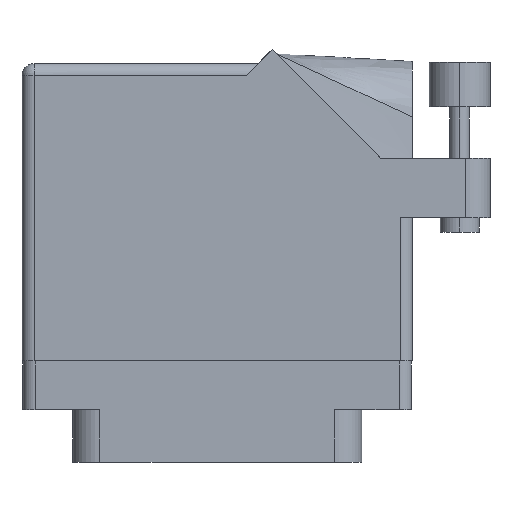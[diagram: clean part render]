
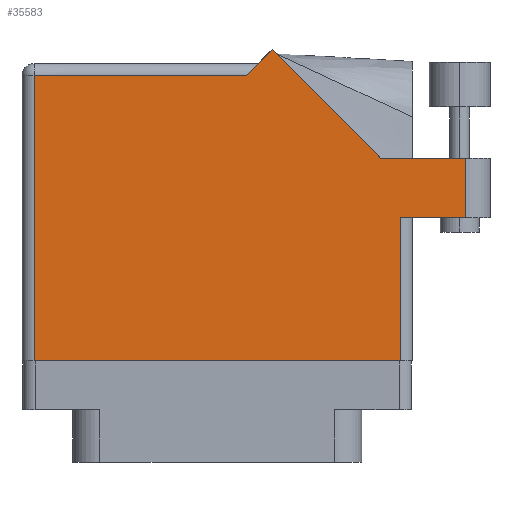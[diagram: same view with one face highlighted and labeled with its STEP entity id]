
A CAD part, front view. The second image highlights one B-rep face of the part: STEP entity #35583.
In plain terms, the highlighted face is planar.
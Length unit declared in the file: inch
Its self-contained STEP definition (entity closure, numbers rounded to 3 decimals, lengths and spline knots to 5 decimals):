
#87 = DIRECTION ( 'NONE',  ( -1., 0., 0. ) ) ;
#300 = LINE ( 'NONE', #7329, #24097 ) ;
#316 = DIRECTION ( 'NONE',  ( 1., 0., 0. ) ) ;
#977 = PLANE ( 'NONE',  #6556 ) ;
#1497 = LINE ( 'NONE', #14227, #21332 ) ;
#1553 = LINE ( 'NONE', #28286, #30628 ) ;
#1587 = EDGE_CURVE ( 'NONE', #17479, #24316, #30932, .T. ) ;
#1897 = ORIENTED_EDGE ( 'NONE', *, *, #10935, .T. ) ;
#1936 = ORIENTED_EDGE ( 'NONE', *, *, #35250, .T. ) ;
#4389 = VECTOR ( 'NONE', #36227, 39.37008 ) ;
#5711 = CARTESIAN_POINT ( 'NONE',  ( 0.83942, 0.944, 0.455 ) ) ;
#5885 = LINE ( 'NONE', #14596, #4389 ) ;
#6556 = AXIS2_PLACEMENT_3D ( 'NONE', #22632, #25769, #38970 ) ;
#7041 = EDGE_CURVE ( 'NONE', #25295, #24932, #35793, .T. ) ;
#7329 = CARTESIAN_POINT ( 'NONE',  ( 1.405, 0.944, 0.455 ) ) ;
#8422 = ORIENTED_EDGE ( 'NONE', *, *, #7041, .T. ) ;
#8563 = LINE ( 'NONE', #26989, #35157 ) ;
#9978 = ORIENTED_EDGE ( 'NONE', *, *, #16870, .T. ) ;
#10122 = ORIENTED_EDGE ( 'NONE', *, *, #39444, .T. ) ;
#10469 = FACE_OUTER_BOUND ( 'NONE', #15278, .T. ) ;
#10810 = DIRECTION ( 'NONE',  ( -0.707, 0.707, 0. ) ) ;
#10935 = EDGE_CURVE ( 'NONE', #15507, #30508, #1553, .T. ) ;
#11664 = CARTESIAN_POINT ( 'NONE',  ( 1.28, 0.637, 0.455 ) ) ;
#11964 = LINE ( 'NONE', #18461, #35651 ) ;
#12001 = DIRECTION ( 'NONE',  ( 0., 1., 0. ) ) ;
#12781 = CARTESIAN_POINT ( 'NONE',  ( 0.943, 0.637, 0.455 ) ) ;
#13068 = VECTOR ( 'NONE', #87, 39.37008 ) ;
#13102 = ORIENTED_EDGE ( 'NONE', *, *, #14538, .T. ) ;
#13276 = CARTESIAN_POINT ( 'NONE',  ( 0.28271, 1.50071, 0.455 ) ) ;
#14227 = CARTESIAN_POINT ( 'NONE',  ( -0.943, -0.1, 0.455 ) ) ;
#14538 = EDGE_CURVE ( 'NONE', #24932, #17479, #1497, .T. ) ;
#14596 = CARTESIAN_POINT ( 'NONE',  ( 0.212, 1.43, 0.455 ) ) ;
#14768 = DIRECTION ( 'NONE',  ( 0., -1., 0. ) ) ;
#15278 = EDGE_LOOP ( 'NONE', ( #39815, #1897, #9978, #10122, #18293, #8422, #13102, #37050, #1936 ) ) ;
#15507 = VERTEX_POINT ( 'NONE', #11664 ) ;
#16870 = EDGE_CURVE ( 'NONE', #30508, #20123, #300, .T. ) ;
#17025 = EDGE_CURVE ( 'NONE', #35901, #25295, #5885, .T. ) ;
#17479 = VERTEX_POINT ( 'NONE', #33991 ) ;
#17503 = DIRECTION ( 'NONE',  ( 1., 0., 0. ) ) ;
#18293 = ORIENTED_EDGE ( 'NONE', *, *, #17025, .T. ) ;
#18461 = CARTESIAN_POINT ( 'NONE',  ( 0.943, 0.637, 0.455 ) ) ;
#18720 = CARTESIAN_POINT ( 'NONE',  ( -0.943, 1.368, 0.455 ) ) ;
#20123 = VERTEX_POINT ( 'NONE', #5711 ) ;
#20669 = LINE ( 'NONE', #38901, #37548 ) ;
#21332 = VECTOR ( 'NONE', #14768, 39.37008 ) ;
#21971 = CARTESIAN_POINT ( 'NONE',  ( -1.005, -0.1, 0.455 ) ) ;
#22632 = CARTESIAN_POINT ( 'NONE',  ( -1.005, 1.43, 0.455 ) ) ;
#22704 = EDGE_CURVE ( 'NONE', #37985, #15507, #8563, .T. ) ;
#24097 = VECTOR ( 'NONE', #25970, 39.37008 ) ;
#24316 = VERTEX_POINT ( 'NONE', #26575 ) ;
#24932 = VERTEX_POINT ( 'NONE', #18720 ) ;
#25284 = CARTESIAN_POINT ( 'NONE',  ( -1.005, 1.368, 0.455 ) ) ;
#25295 = VERTEX_POINT ( 'NONE', #26430 ) ;
#25601 = VECTOR ( 'NONE', #316, 39.37008 ) ;
#25769 = DIRECTION ( 'NONE',  ( 0., 0., -1. ) ) ;
#25970 = DIRECTION ( 'NONE',  ( -1., 0., 0. ) ) ;
#26430 = CARTESIAN_POINT ( 'NONE',  ( 0.15, 1.368, 0.455 ) ) ;
#26575 = CARTESIAN_POINT ( 'NONE',  ( 0.943, -0.1, 0.455 ) ) ;
#26989 = CARTESIAN_POINT ( 'NONE',  ( 1.005, 0.637, 0.455 ) ) ;
#28286 = CARTESIAN_POINT ( 'NONE',  ( 1.28, 0.944, 0.455 ) ) ;
#30508 = VERTEX_POINT ( 'NONE', #39929 ) ;
#30628 = VECTOR ( 'NONE', #35158, 39.37008 ) ;
#30932 = LINE ( 'NONE', #21971, #25601 ) ;
#33991 = CARTESIAN_POINT ( 'NONE',  ( -0.943, -0.1, 0.455 ) ) ;
#35157 = VECTOR ( 'NONE', #17503, 39.37008 ) ;
#35158 = DIRECTION ( 'NONE',  ( 0., 1., 0. ) ) ;
#35250 = EDGE_CURVE ( 'NONE', #24316, #37985, #11964, .T. ) ;
#35583 = ADVANCED_FACE ( 'NONE', ( #10469 ), #977, .F. ) ;
#35651 = VECTOR ( 'NONE', #12001, 39.37008 ) ;
#35793 = LINE ( 'NONE', #25284, #13068 ) ;
#35901 = VERTEX_POINT ( 'NONE', #13276 ) ;
#36227 = DIRECTION ( 'NONE',  ( -0.707, -0.707, 0. ) ) ;
#37050 = ORIENTED_EDGE ( 'NONE', *, *, #1587, .T. ) ;
#37548 = VECTOR ( 'NONE', #10810, 39.37008 ) ;
#37985 = VERTEX_POINT ( 'NONE', #12781 ) ;
#38901 = CARTESIAN_POINT ( 'NONE',  ( 0.83942, 0.944, 0.455 ) ) ;
#38970 = DIRECTION ( 'NONE',  ( -1., 0., 0. ) ) ;
#39444 = EDGE_CURVE ( 'NONE', #20123, #35901, #20669, .T. ) ;
#39815 = ORIENTED_EDGE ( 'NONE', *, *, #22704, .T. ) ;
#39929 = CARTESIAN_POINT ( 'NONE',  ( 1.28, 0.944, 0.455 ) ) ;
